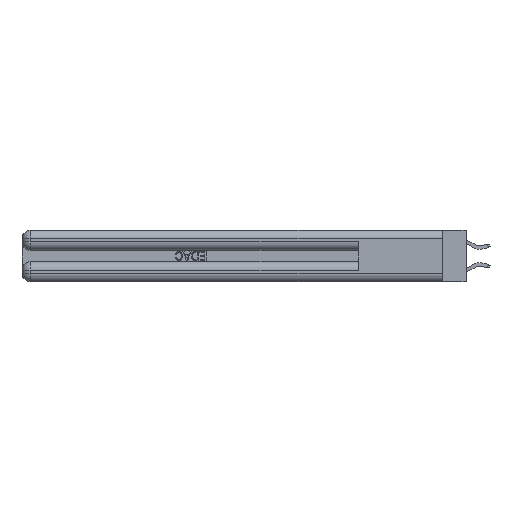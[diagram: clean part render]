
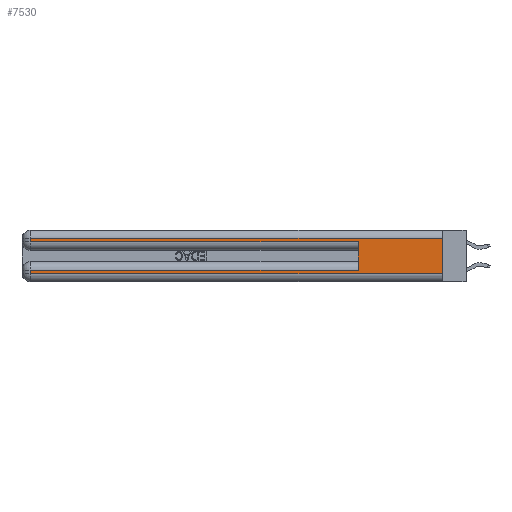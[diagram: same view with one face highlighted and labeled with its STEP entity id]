
A CAD part, left-side view. The second image highlights one B-rep face of the part: STEP entity #7530.
In plain terms, the highlighted planar face has unit normal (-1, 0, 0).
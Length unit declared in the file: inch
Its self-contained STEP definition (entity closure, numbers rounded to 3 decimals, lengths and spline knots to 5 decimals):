
#1031 = CARTESIAN_POINT ( 'NONE',  ( 0., 0., 0.285 ) ) ;
#1194 = LINE ( 'NONE', #1031, #6302 ) ;
#2157 = DIRECTION ( 'NONE',  ( 0., 1., 0. ) ) ;
#2436 = CARTESIAN_POINT ( 'NONE',  ( 0., 0.6, 0.285 ) ) ;
#2909 = CARTESIAN_POINT ( 'NONE',  ( 0., 2.94, 0.37 ) ) ;
#2949 = DIRECTION ( 'NONE',  ( 0., 0., -1. ) ) ;
#3057 = DIRECTION ( 'NONE',  ( 0., 0., -1. ) ) ;
#3935 = ORIENTED_EDGE ( 'NONE', *, *, #9410, .T. ) ;
#4792 = CARTESIAN_POINT ( 'NONE',  ( 0., 0., 0.37 ) ) ;
#5312 = ORIENTED_EDGE ( 'NONE', *, *, #6509, .T. ) ;
#5334 = FACE_OUTER_BOUND ( 'NONE', #12879, .T. ) ;
#5437 = CARTESIAN_POINT ( 'NONE',  ( 0., 2.94, 0.31 ) ) ;
#6302 = VECTOR ( 'NONE', #14808, 39.37008 ) ;
#6413 = CARTESIAN_POINT ( 'NONE',  ( 0., 2.94, 0.085 ) ) ;
#6509 = EDGE_CURVE ( 'NONE', #21605, #12849, #15656, .T. ) ;
#7184 = LINE ( 'NONE', #9276, #18147 ) ;
#7530 = ADVANCED_FACE ( 'NONE', ( #5334 ), #23357, .F. ) ;
#8955 = VECTOR ( 'NONE', #3057, 39.37008 ) ;
#9140 = EDGE_CURVE ( 'NONE', #22862, #24134, #19070, .T. ) ;
#9259 = VERTEX_POINT ( 'NONE', #2436 ) ;
#9276 = CARTESIAN_POINT ( 'NONE',  ( 0., 0., 0.085 ) ) ;
#9410 = EDGE_CURVE ( 'NONE', #20529, #12989, #7184, .T. ) ;
#9849 = ORIENTED_EDGE ( 'NONE', *, *, #16280, .T. ) ;
#10375 = CARTESIAN_POINT ( 'NONE',  ( 0., 0., 0.06 ) ) ;
#10897 = CARTESIAN_POINT ( 'NONE',  ( 0., 0., 0.31 ) ) ;
#11617 = DIRECTION ( 'NONE',  ( 0., 0., -1. ) ) ;
#12024 = CARTESIAN_POINT ( 'NONE',  ( 0., 0.6, 0.085 ) ) ;
#12334 = EDGE_CURVE ( 'NONE', #13108, #21605, #28621, .T. ) ;
#12492 = ORIENTED_EDGE ( 'NONE', *, *, #16512, .F. ) ;
#12642 = CARTESIAN_POINT ( 'NONE',  ( 0., 0.6, 0.145 ) ) ;
#12849 = VERTEX_POINT ( 'NONE', #19558 ) ;
#12872 = ORIENTED_EDGE ( 'NONE', *, *, #17959, .F. ) ;
#12879 = EDGE_LOOP ( 'NONE', ( #12872, #20689, #5312, #28318, #12492, #3935, #9849, #22667 ) ) ;
#12989 = VERTEX_POINT ( 'NONE', #6413 ) ;
#13108 = VERTEX_POINT ( 'NONE', #14745 ) ;
#13740 = CARTESIAN_POINT ( 'NONE',  ( 0., 0., 0.06 ) ) ;
#14745 = CARTESIAN_POINT ( 'NONE',  ( 0., 0., 0.31 ) ) ;
#14808 = DIRECTION ( 'NONE',  ( 0., -1., 0. ) ) ;
#15418 = VECTOR ( 'NONE', #23124, 39.37008 ) ;
#15656 = LINE ( 'NONE', #2909, #8955 ) ;
#16280 = EDGE_CURVE ( 'NONE', #12989, #22862, #19308, .T. ) ;
#16512 = EDGE_CURVE ( 'NONE', #20529, #9259, #26239, .T. ) ;
#17959 = EDGE_CURVE ( 'NONE', #13108, #24134, #18252, .T. ) ;
#18147 = VECTOR ( 'NONE', #2157, 39.37008 ) ;
#18171 = VECTOR ( 'NONE', #28094, 39.37008 ) ;
#18252 = LINE ( 'NONE', #4792, #24755 ) ;
#18638 = DIRECTION ( 'NONE',  ( 1., 0., 0. ) ) ;
#18896 = CARTESIAN_POINT ( 'NONE',  ( 0., 2.94, 0.06 ) ) ;
#19070 = LINE ( 'NONE', #10375, #18171 ) ;
#19308 = LINE ( 'NONE', #28323, #15418 ) ;
#19558 = CARTESIAN_POINT ( 'NONE',  ( 0., 2.94, 0.285 ) ) ;
#20020 = DIRECTION ( 'NONE',  ( 0., 0., 1. ) ) ;
#20529 = VERTEX_POINT ( 'NONE', #12024 ) ;
#20689 = ORIENTED_EDGE ( 'NONE', *, *, #12334, .T. ) ;
#21016 = CARTESIAN_POINT ( 'NONE',  ( 0., 0., 0.37 ) ) ;
#21605 = VERTEX_POINT ( 'NONE', #5437 ) ;
#21805 = DIRECTION ( 'NONE',  ( 0., 1., 0. ) ) ;
#22185 = AXIS2_PLACEMENT_3D ( 'NONE', #21016, #18638, #2949 ) ;
#22667 = ORIENTED_EDGE ( 'NONE', *, *, #9140, .T. ) ;
#22862 = VERTEX_POINT ( 'NONE', #18896 ) ;
#23124 = DIRECTION ( 'NONE',  ( 0., 0., -1. ) ) ;
#23357 = PLANE ( 'NONE',  #22185 ) ;
#24134 = VERTEX_POINT ( 'NONE', #13740 ) ;
#24755 = VECTOR ( 'NONE', #11617, 39.37008 ) ;
#26239 = LINE ( 'NONE', #12642, #27318 ) ;
#27318 = VECTOR ( 'NONE', #20020, 39.37008 ) ;
#27559 = VECTOR ( 'NONE', #21805, 39.37008 ) ;
#27611 = EDGE_CURVE ( 'NONE', #12849, #9259, #1194, .T. ) ;
#28094 = DIRECTION ( 'NONE',  ( 0., -1., 0. ) ) ;
#28318 = ORIENTED_EDGE ( 'NONE', *, *, #27611, .T. ) ;
#28323 = CARTESIAN_POINT ( 'NONE',  ( 0., 2.94, 0.37 ) ) ;
#28621 = LINE ( 'NONE', #10897, #27559 ) ;
